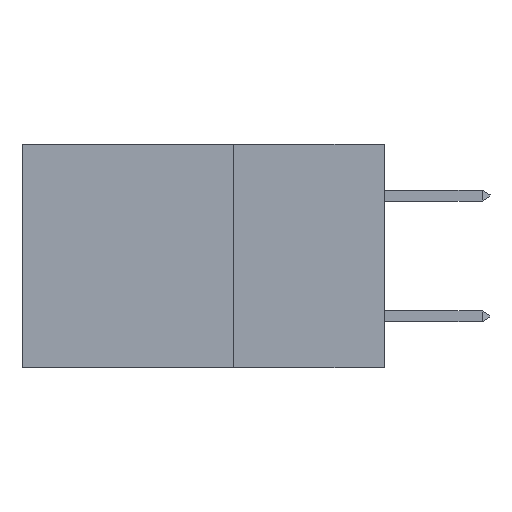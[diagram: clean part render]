
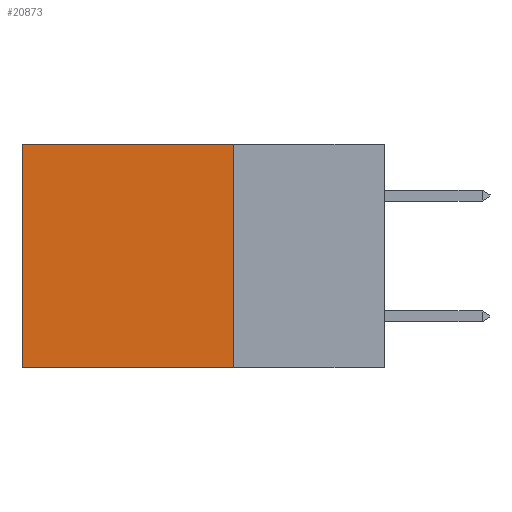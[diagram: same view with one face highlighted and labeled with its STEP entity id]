
A CAD part, left-side view. The second image highlights one B-rep face of the part: STEP entity #20873.
In plain terms, the highlighted planar face has unit normal (-1, 0, 0).
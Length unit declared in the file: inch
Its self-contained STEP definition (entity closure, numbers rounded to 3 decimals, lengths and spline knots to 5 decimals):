
#102 = AXIS2_PLACEMENT_3D ( 'NONE', #34598, #14246, #37986 ) ;
#861 = VECTOR ( 'NONE', #1779, 39.37008 ) ;
#1779 = DIRECTION ( 'NONE',  ( 0., 1., 0. ) ) ;
#2884 = ORIENTED_EDGE ( 'NONE', *, *, #15069, .F. ) ;
#3668 = LINE ( 'NONE', #40687, #38781 ) ;
#3761 = EDGE_LOOP ( 'NONE', ( #15859, #2884, #37271, #42288 ) ) ;
#5289 = DIRECTION ( 'NONE',  ( 0., 0., -1. ) ) ;
#6320 = EDGE_CURVE ( 'NONE', #35479, #42457, #37018, .T. ) ;
#10806 = PLANE ( 'NONE',  #102 ) ;
#12365 = VERTEX_POINT ( 'NONE', #20863 ) ;
#14246 = DIRECTION ( 'NONE',  ( 1., 0., 0. ) ) ;
#14891 = CARTESIAN_POINT ( 'NONE',  ( 0.2875, 0.6, 0. ) ) ;
#15024 = EDGE_CURVE ( 'NONE', #35479, #18193, #42356, .T. ) ;
#15069 = EDGE_CURVE ( 'NONE', #18193, #12365, #40212, .T. ) ;
#15859 = ORIENTED_EDGE ( 'NONE', *, *, #34162, .T. ) ;
#18193 = VERTEX_POINT ( 'NONE', #26128 ) ;
#18785 = CARTESIAN_POINT ( 'NONE',  ( 0.2875, 0.25, 0. ) ) ;
#20863 = CARTESIAN_POINT ( 'NONE',  ( 0.2875, 0.6, -0.37 ) ) ;
#20873 = ADVANCED_FACE ( 'NONE', ( #24443 ), #10806, .F. ) ;
#22597 = CARTESIAN_POINT ( 'NONE',  ( 0.2875, 0.25, 0. ) ) ;
#24443 = FACE_OUTER_BOUND ( 'NONE', #3761, .T. ) ;
#26011 = CARTESIAN_POINT ( 'NONE',  ( 0.2875, 0.25, -0.37 ) ) ;
#26128 = CARTESIAN_POINT ( 'NONE',  ( 0.2875, 0.25, -0.37 ) ) ;
#27243 = DIRECTION ( 'NONE',  ( 0., 0., -1. ) ) ;
#29411 = DIRECTION ( 'NONE',  ( 0., 1., 0. ) ) ;
#32299 = VECTOR ( 'NONE', #5289, 39.37008 ) ;
#34162 = EDGE_CURVE ( 'NONE', #42457, #12365, #3668, .T. ) ;
#34598 = CARTESIAN_POINT ( 'NONE',  ( 0.2875, 0.25, 0. ) ) ;
#35479 = VERTEX_POINT ( 'NONE', #22597 ) ;
#35917 = CARTESIAN_POINT ( 'NONE',  ( 0.2875, 0.25, 0. ) ) ;
#37018 = LINE ( 'NONE', #18785, #861 ) ;
#37271 = ORIENTED_EDGE ( 'NONE', *, *, #15024, .F. ) ;
#37986 = DIRECTION ( 'NONE',  ( 0., 0., -1. ) ) ;
#38781 = VECTOR ( 'NONE', #27243, 39.37008 ) ;
#39164 = VECTOR ( 'NONE', #29411, 39.37008 ) ;
#40212 = LINE ( 'NONE', #26011, #39164 ) ;
#40687 = CARTESIAN_POINT ( 'NONE',  ( 0.2875, 0.6, 0. ) ) ;
#42288 = ORIENTED_EDGE ( 'NONE', *, *, #6320, .T. ) ;
#42356 = LINE ( 'NONE', #35917, #32299 ) ;
#42457 = VERTEX_POINT ( 'NONE', #14891 ) ;
